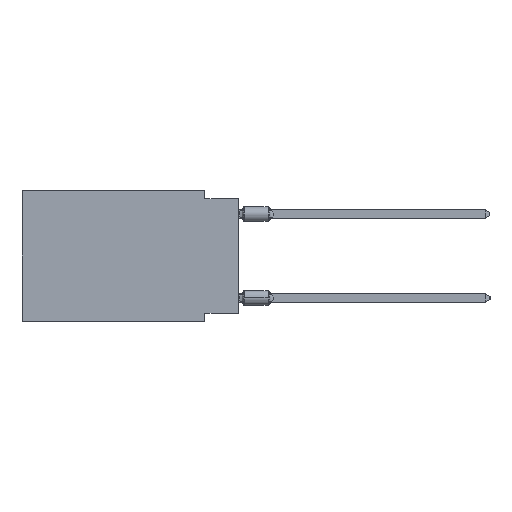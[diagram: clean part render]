
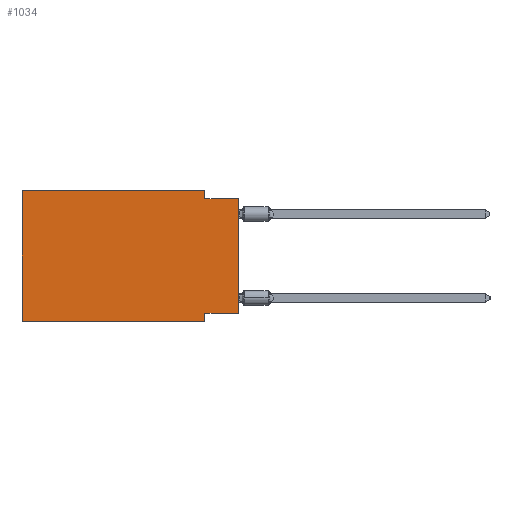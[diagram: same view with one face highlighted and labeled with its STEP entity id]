
A CAD part, left-side view. The second image highlights one B-rep face of the part: STEP entity #1034.
In plain terms, the highlighted planar face has unit normal (-1, 0, 0).
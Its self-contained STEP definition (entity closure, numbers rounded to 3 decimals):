
#160 = ORIENTED_EDGE ( 'NONE', *, *, #18623, .F. ) ;
#472 = ORIENTED_EDGE ( 'NONE', *, *, #28156, .F. ) ;
#494 = VERTEX_POINT ( 'NONE', #37173 ) ;
#1034 = ADVANCED_FACE ( 'NONE', ( #28838 ), #5554, .F. ) ;
#4105 = VECTOR ( 'NONE', #35245, 1000. ) ;
#4736 = ORIENTED_EDGE ( 'NONE', *, *, #24670, .T. ) ;
#5554 = PLANE ( 'NONE',  #20816 ) ;
#5842 = ORIENTED_EDGE ( 'NONE', *, *, #22397, .F. ) ;
#8835 = LINE ( 'NONE', #31533, #17172 ) ;
#11092 = VECTOR ( 'NONE', #49335, 1000. ) ;
#13102 = VERTEX_POINT ( 'NONE', #52744 ) ;
#14137 = DIRECTION ( 'NONE',  ( 1., 0., 0. ) ) ;
#16385 = CARTESIAN_POINT ( 'NONE',  ( 0., 2.54, -0.635 ) ) ;
#16464 = CARTESIAN_POINT ( 'NONE',  ( 0., 0., 0. ) ) ;
#17172 = VECTOR ( 'NONE', #27526, 1000. ) ;
#18623 = EDGE_CURVE ( 'NONE', #25112, #33158, #38415, .T. ) ;
#20219 = CARTESIAN_POINT ( 'NONE',  ( 0., 0., -0.635 ) ) ;
#20816 = AXIS2_PLACEMENT_3D ( 'NONE', #37453, #14137, #51866 ) ;
#21729 = CARTESIAN_POINT ( 'NONE',  ( 0., 16.383, 0. ) ) ;
#22397 = EDGE_CURVE ( 'NONE', #40782, #37831, #40616, .T. ) ;
#23912 = LINE ( 'NONE', #58478, #41255 ) ;
#24575 = EDGE_CURVE ( 'NONE', #13102, #25112, #8835, .T. ) ;
#24670 = EDGE_CURVE ( 'NONE', #42683, #33158, #60057, .T. ) ;
#24827 = VECTOR ( 'NONE', #58738, 1000. ) ;
#25112 = VERTEX_POINT ( 'NONE', #49874 ) ;
#25354 = DIRECTION ( 'NONE',  ( 0., -1., 0. ) ) ;
#26614 = CARTESIAN_POINT ( 'NONE',  ( 0., 2.54, -9.906 ) ) ;
#26791 = VECTOR ( 'NONE', #53270, 1000. ) ;
#26916 = VECTOR ( 'NONE', #50550, 1000. ) ;
#27526 = DIRECTION ( 'NONE',  ( 0., 1., 0. ) ) ;
#28156 = EDGE_CURVE ( 'NONE', #494, #40782, #35043, .T. ) ;
#28838 = FACE_OUTER_BOUND ( 'NONE', #38581, .T. ) ;
#30591 = CARTESIAN_POINT ( 'NONE',  ( 0., 16.383, -9.906 ) ) ;
#30595 = ORIENTED_EDGE ( 'NONE', *, *, #50160, .F. ) ;
#31533 = CARTESIAN_POINT ( 'NONE',  ( 0., 0., -9.271 ) ) ;
#32535 = CARTESIAN_POINT ( 'NONE',  ( 0., 2.54, 0. ) ) ;
#33158 = VERTEX_POINT ( 'NONE', #26614 ) ;
#35043 = LINE ( 'NONE', #44537, #45689 ) ;
#35245 = DIRECTION ( 'NONE',  ( 0., 0., -1. ) ) ;
#35339 = DIRECTION ( 'NONE',  ( 0., -1., 0. ) ) ;
#35759 = LINE ( 'NONE', #16464, #26791 ) ;
#37173 = CARTESIAN_POINT ( 'NONE',  ( 0., 16.383, 0. ) ) ;
#37453 = CARTESIAN_POINT ( 'NONE',  ( 0., 16.383, 0. ) ) ;
#37831 = VERTEX_POINT ( 'NONE', #16385 ) ;
#38415 = LINE ( 'NONE', #54245, #4105 ) ;
#38581 = EDGE_LOOP ( 'NONE', ( #39518, #59647, #5842, #472, #30595, #4736, #160, #52229 ) ) ;
#39518 = ORIENTED_EDGE ( 'NONE', *, *, #50623, .T. ) ;
#40616 = LINE ( 'NONE', #44926, #24827 ) ;
#40782 = VERTEX_POINT ( 'NONE', #32535 ) ;
#41255 = VECTOR ( 'NONE', #25354, 1000. ) ;
#42683 = VERTEX_POINT ( 'NONE', #30591 ) ;
#44537 = CARTESIAN_POINT ( 'NONE',  ( 0., 16.383, 0. ) ) ;
#44737 = LINE ( 'NONE', #21729, #11092 ) ;
#44760 = VERTEX_POINT ( 'NONE', #20219 ) ;
#44926 = CARTESIAN_POINT ( 'NONE',  ( 0., 2.54, 0. ) ) ;
#45689 = VECTOR ( 'NONE', #35339, 1000. ) ;
#45939 = CARTESIAN_POINT ( 'NONE',  ( 0., 16.383, -9.906 ) ) ;
#48819 = EDGE_CURVE ( 'NONE', #37831, #44760, #23912, .T. ) ;
#49335 = DIRECTION ( 'NONE',  ( 0., 0., 1. ) ) ;
#49874 = CARTESIAN_POINT ( 'NONE',  ( 0., 2.54, -9.271 ) ) ;
#50160 = EDGE_CURVE ( 'NONE', #42683, #494, #44737, .T. ) ;
#50550 = DIRECTION ( 'NONE',  ( 0., -1., 0. ) ) ;
#50623 = EDGE_CURVE ( 'NONE', #13102, #44760, #35759, .T. ) ;
#51866 = DIRECTION ( 'NONE',  ( 0., 0., -1. ) ) ;
#52229 = ORIENTED_EDGE ( 'NONE', *, *, #24575, .F. ) ;
#52744 = CARTESIAN_POINT ( 'NONE',  ( 0., 0., -9.271 ) ) ;
#53270 = DIRECTION ( 'NONE',  ( 0., 0., 1. ) ) ;
#54245 = CARTESIAN_POINT ( 'NONE',  ( 0., 2.54, -9.906 ) ) ;
#58478 = CARTESIAN_POINT ( 'NONE',  ( 0., 0., -0.635 ) ) ;
#58738 = DIRECTION ( 'NONE',  ( 0., 0., -1. ) ) ;
#59647 = ORIENTED_EDGE ( 'NONE', *, *, #48819, .F. ) ;
#60057 = LINE ( 'NONE', #45939, #26916 ) ;
